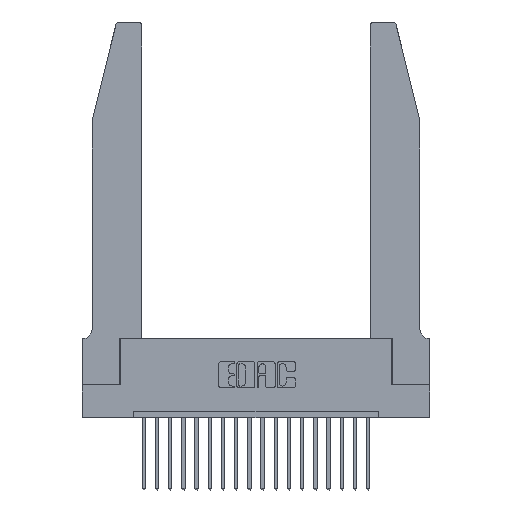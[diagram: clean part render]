
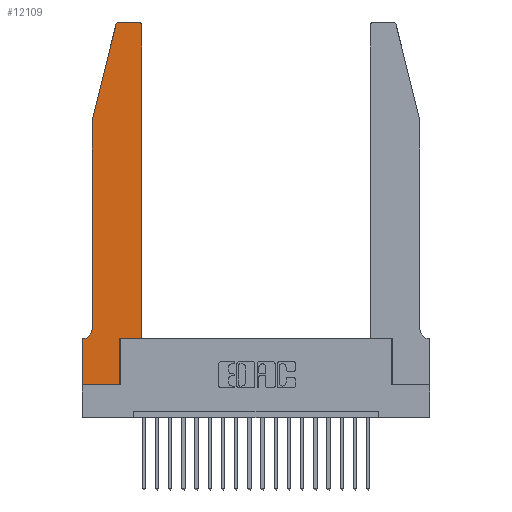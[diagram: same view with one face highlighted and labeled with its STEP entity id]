
A CAD part, top view. The second image highlights one B-rep face of the part: STEP entity #12109.
In plain terms, the highlighted planar face has unit normal (0, 0, 1).
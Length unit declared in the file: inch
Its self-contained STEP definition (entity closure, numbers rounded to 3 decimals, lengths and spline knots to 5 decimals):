
#290 = CARTESIAN_POINT ( 'NONE',  ( 0.0755, 2., 0.37 ) ) ;
#887 = CARTESIAN_POINT ( 'NONE',  ( 0.0055, 0.35, 0.37 ) ) ;
#921 = EDGE_CURVE ( 'NONE', #10105, #7049, #10771, .T. ) ;
#936 = AXIS2_PLACEMENT_3D ( 'NONE', #8221, #19752, #8289 ) ;
#987 = EDGE_CURVE ( 'NONE', #8814, #12497, #10494, .T. ) ;
#1107 = ORIENTED_EDGE ( 'NONE', *, *, #921, .T. ) ;
#1275 = ORIENTED_EDGE ( 'NONE', *, *, #12326, .T. ) ;
#1502 = LINE ( 'NONE', #14445, #20977 ) ;
#1570 = LINE ( 'NONE', #16977, #13751 ) ;
#1591 = ORIENTED_EDGE ( 'NONE', *, *, #7726, .T. ) ;
#1811 = DIRECTION ( 'NONE',  ( 0., 0., -1. ) ) ;
#2357 = ORIENTED_EDGE ( 'NONE', *, *, #17164, .T. ) ;
#2386 = DIRECTION ( 'NONE',  ( 1., 0., 0. ) ) ;
#2706 = CARTESIAN_POINT ( 'NONE',  ( 0.284, 2.75, 0.37 ) ) ;
#3595 = EDGE_CURVE ( 'NONE', #13025, #21496, #10011, .T. ) ;
#3613 = LINE ( 'NONE', #18891, #3851 ) ;
#3851 = VECTOR ( 'NONE', #8945, 39.37008 ) ;
#4242 = FACE_OUTER_BOUND ( 'NONE', #15336, .T. ) ;
#4947 = DIRECTION ( 'NONE',  ( -1., 0., 0. ) ) ;
#5014 = ORIENTED_EDGE ( 'NONE', *, *, #14510, .T. ) ;
#5156 = CARTESIAN_POINT ( 'NONE',  ( 0.2865, 0., 0.37 ) ) ;
#5418 = AXIS2_PLACEMENT_3D ( 'NONE', #12161, #13900, #2386 ) ;
#5665 = DIRECTION ( 'NONE',  ( 1., 0., 0. ) ) ;
#6313 = VECTOR ( 'NONE', #20181, 39.37008 ) ;
#6343 = ORIENTED_EDGE ( 'NONE', *, *, #8678, .T. ) ;
#6384 = CARTESIAN_POINT ( 'NONE',  ( 0.0755, 2., 0.37 ) ) ;
#6842 = VECTOR ( 'NONE', #14543, 39.37008 ) ;
#6891 = ORIENTED_EDGE ( 'NONE', *, *, #12356, .T. ) ;
#7049 = VERTEX_POINT ( 'NONE', #16444 ) ;
#7130 = ORIENTED_EDGE ( 'NONE', *, *, #17266, .T. ) ;
#7424 = CARTESIAN_POINT ( 'NONE',  ( 0.25487, 2.72718, 0.37 ) ) ;
#7726 = EDGE_CURVE ( 'NONE', #12497, #17196, #12389, .T. ) ;
#8006 = CARTESIAN_POINT ( 'NONE',  ( 0.4505, 0.35, 0.37 ) ) ;
#8066 = CARTESIAN_POINT ( 'NONE',  ( 0.0755, 2., 0.37 ) ) ;
#8105 = AXIS2_PLACEMENT_3D ( 'NONE', #15106, #1811, #4947 ) ;
#8150 = EDGE_CURVE ( 'NONE', #19930, #10105, #18933, .T. ) ;
#8221 = CARTESIAN_POINT ( 'NONE',  ( 0.4205, 2.72, 0.37 ) ) ;
#8289 = DIRECTION ( 'NONE',  ( 1., 0., 0. ) ) ;
#8678 = EDGE_CURVE ( 'NONE', #14540, #19930, #1502, .T. ) ;
#8814 = VERTEX_POINT ( 'NONE', #15974 ) ;
#8945 = DIRECTION ( 'NONE',  ( -1., 0., 0. ) ) ;
#9190 = EDGE_CURVE ( 'NONE', #9591, #15513, #18373, .T. ) ;
#9591 = VERTEX_POINT ( 'NONE', #10584 ) ;
#9643 = DIRECTION ( 'NONE',  ( 1., 0., 0. ) ) ;
#9815 = CARTESIAN_POINT ( 'NONE',  ( 0., 0., 0.37 ) ) ;
#10011 = CIRCLE ( 'NONE', #5418, 0.03 ) ;
#10105 = VERTEX_POINT ( 'NONE', #10394 ) ;
#10363 = DIRECTION ( 'NONE',  ( -1., 0., 0. ) ) ;
#10394 = CARTESIAN_POINT ( 'NONE',  ( 0.4505, 2.72, 0.37 ) ) ;
#10494 = LINE ( 'NONE', #9815, #13336 ) ;
#10584 = CARTESIAN_POINT ( 'NONE',  ( 0.0755, 0.42, 0.37 ) ) ;
#10718 = LINE ( 'NONE', #290, #6313 ) ;
#10771 = CIRCLE ( 'NONE', #936, 0.03 ) ;
#11177 = LINE ( 'NONE', #14887, #18467 ) ;
#11263 = VERTEX_POINT ( 'NONE', #6384 ) ;
#12109 = ADVANCED_FACE ( 'NONE', ( #4242 ), #13679, .T. ) ;
#12161 = CARTESIAN_POINT ( 'NONE',  ( 0.284, 2.72, 0.37 ) ) ;
#12197 = CARTESIAN_POINT ( 'NONE',  ( 0.2865, 0.35, 0.37 ) ) ;
#12326 = EDGE_CURVE ( 'NONE', #21496, #11263, #14100, .T. ) ;
#12356 = EDGE_CURVE ( 'NONE', #11263, #9591, #10718, .T. ) ;
#12389 = LINE ( 'NONE', #15316, #20188 ) ;
#12497 = VERTEX_POINT ( 'NONE', #17935 ) ;
#13025 = VERTEX_POINT ( 'NONE', #2706 ) ;
#13336 = VECTOR ( 'NONE', #19829, 39.37008 ) ;
#13679 = PLANE ( 'NONE',  #18448 ) ;
#13751 = VECTOR ( 'NONE', #10363, 39.37008 ) ;
#13900 = DIRECTION ( 'NONE',  ( 0., 0., 1. ) ) ;
#14100 = LINE ( 'NONE', #8066, #6842 ) ;
#14445 = CARTESIAN_POINT ( 'NONE',  ( 0.4505, 0.35, 0.37 ) ) ;
#14510 = EDGE_CURVE ( 'NONE', #15513, #8814, #3613, .T. ) ;
#14540 = VERTEX_POINT ( 'NONE', #12197 ) ;
#14543 = DIRECTION ( 'NONE',  ( -0.239, -0.971, 0. ) ) ;
#14887 = CARTESIAN_POINT ( 'NONE',  ( 0.2865, 0.35, 0.37 ) ) ;
#15106 = CARTESIAN_POINT ( 'NONE',  ( 0.0055, 0.42, 0.37 ) ) ;
#15314 = ORIENTED_EDGE ( 'NONE', *, *, #8150, .T. ) ;
#15316 = CARTESIAN_POINT ( 'NONE',  ( 0., 0., 0.37 ) ) ;
#15336 = EDGE_LOOP ( 'NONE', ( #7130, #21226, #1275, #6891, #17436, #5014, #15351, #1591, #2357, #6343, #15314, #1107 ) ) ;
#15351 = ORIENTED_EDGE ( 'NONE', *, *, #987, .T. ) ;
#15513 = VERTEX_POINT ( 'NONE', #887 ) ;
#15578 = DIRECTION ( 'NONE',  ( 0., 0., 1. ) ) ;
#15974 = CARTESIAN_POINT ( 'NONE',  ( 0., 0.35, 0.37 ) ) ;
#16444 = CARTESIAN_POINT ( 'NONE',  ( 0.4205, 2.75, 0.37 ) ) ;
#16977 = CARTESIAN_POINT ( 'NONE',  ( 0.2605, 2.75, 0.37 ) ) ;
#17113 = DIRECTION ( 'NONE',  ( 1., 0., 0. ) ) ;
#17164 = EDGE_CURVE ( 'NONE', #17196, #14540, #11177, .T. ) ;
#17170 = CARTESIAN_POINT ( 'NONE',  ( 0., 0.35, 0.37 ) ) ;
#17196 = VERTEX_POINT ( 'NONE', #5156 ) ;
#17266 = EDGE_CURVE ( 'NONE', #7049, #13025, #1570, .T. ) ;
#17436 = ORIENTED_EDGE ( 'NONE', *, *, #9190, .T. ) ;
#17635 = DIRECTION ( 'NONE',  ( 0., 1., 0. ) ) ;
#17935 = CARTESIAN_POINT ( 'NONE',  ( 0., 0., 0.37 ) ) ;
#18373 = CIRCLE ( 'NONE', #8105, 0.07 ) ;
#18448 = AXIS2_PLACEMENT_3D ( 'NONE', #17170, #15578, #5665 ) ;
#18467 = VECTOR ( 'NONE', #19882, 39.37008 ) ;
#18891 = CARTESIAN_POINT ( 'NONE',  ( 0.0755, 0.35, 0.37 ) ) ;
#18933 = LINE ( 'NONE', #8006, #19688 ) ;
#19688 = VECTOR ( 'NONE', #17635, 39.37008 ) ;
#19752 = DIRECTION ( 'NONE',  ( 0., 0., 1. ) ) ;
#19829 = DIRECTION ( 'NONE',  ( 0., -1., 0. ) ) ;
#19882 = DIRECTION ( 'NONE',  ( 0., 1., 0. ) ) ;
#19930 = VERTEX_POINT ( 'NONE', #21276 ) ;
#20181 = DIRECTION ( 'NONE',  ( 0., -1., 0. ) ) ;
#20188 = VECTOR ( 'NONE', #17113, 39.37008 ) ;
#20977 = VECTOR ( 'NONE', #9643, 39.37008 ) ;
#21226 = ORIENTED_EDGE ( 'NONE', *, *, #3595, .T. ) ;
#21276 = CARTESIAN_POINT ( 'NONE',  ( 0.4505, 0.35, 0.37 ) ) ;
#21496 = VERTEX_POINT ( 'NONE', #7424 ) ;
